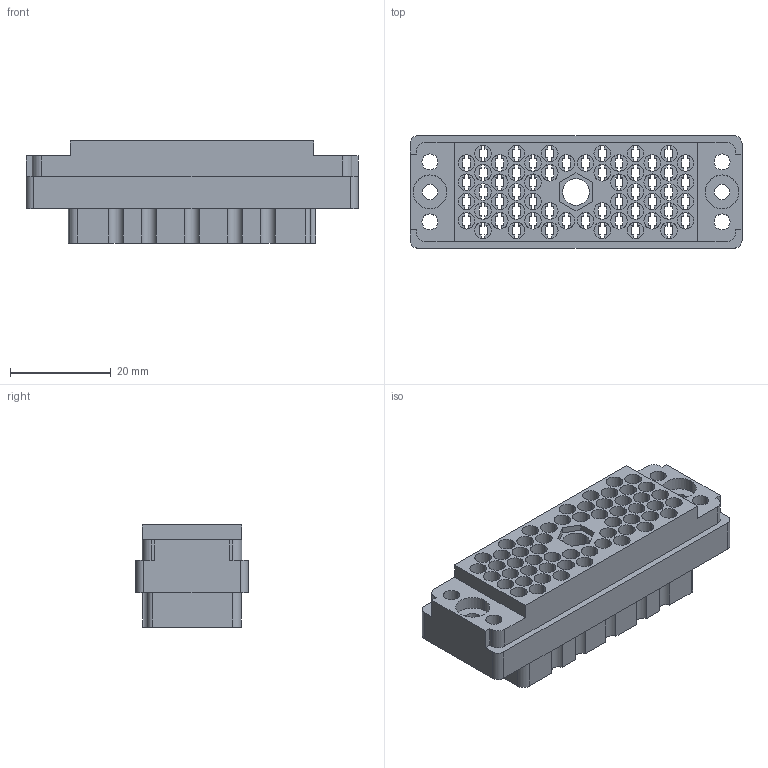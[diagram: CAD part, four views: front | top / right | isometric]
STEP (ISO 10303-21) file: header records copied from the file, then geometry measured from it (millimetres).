
FILE_DESCRIPTION (( 'STEP AP203' ), '1' );
FILE_NAME ('516-056-000-200.STEP', '2020-03-05T19:16:57', ( '' ), ( '' ), 'SwSTEP 2.0', 'SolidWorks 2016', '' );
FILE_SCHEMA (( 'CONFIG_CONTROL_DESIGN' ));
Length unit declared in the file: inch
Products named in the file (2): 516-056-000-200; 516 Part Receptacle_056
Assembly tree (1 placements, depth 2):
  516-056-000-200
    516 Part Receptacle_056
Bounding box: 65.84 x 22.25 x 20.27 mm (x, y, z)
Volume: 13982.3 mm3; surface area: 19760.6 mm2
Topology: 1 solids, 1 shells, 1266 faces, 3740 edges, 2492 vertices
Faces by surface type: plane 893, cylinder 371, cone 2
Entity records: 42750 total; most frequent: CARTESIAN_POINT 7502, ORIENTED_EDGE 7480, DIRECTION 7246, EDGE_CURVE 3740, VECTOR 2774, LINE 2774, VERTEX_POINT 2492, AXIS2_PLACEMENT_3D 2236
